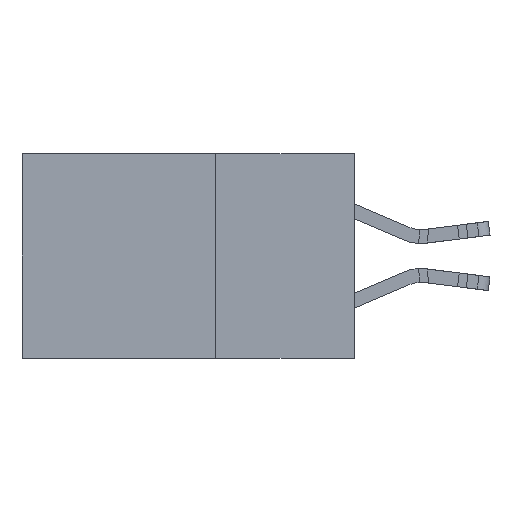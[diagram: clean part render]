
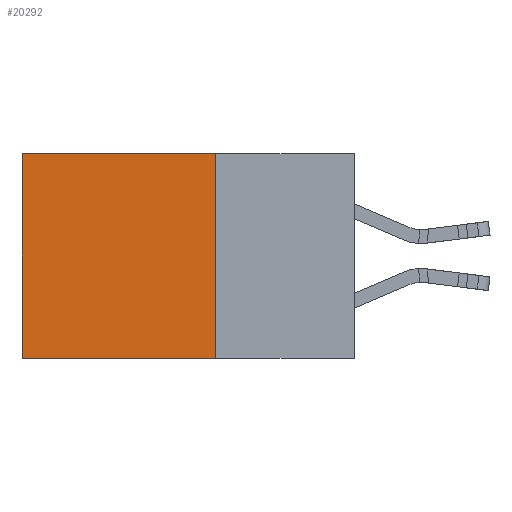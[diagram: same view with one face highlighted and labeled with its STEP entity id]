
A CAD part, left-side view. The second image highlights one B-rep face of the part: STEP entity #20292.
In plain terms, the highlighted planar face has unit normal (-1, 0, 0).
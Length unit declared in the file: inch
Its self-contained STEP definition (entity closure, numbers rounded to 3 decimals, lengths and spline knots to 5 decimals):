
#1641 = DIRECTION ( 'NONE',  ( 0., 1., 0. ) ) ;
#3402 = VERTEX_POINT ( 'NONE', #5823 ) ;
#4192 = EDGE_CURVE ( 'NONE', #12284, #3402, #6441, .T. ) ;
#5823 = CARTESIAN_POINT ( 'NONE',  ( 0.298, 0.6, 0. ) ) ;
#6295 = CARTESIAN_POINT ( 'NONE',  ( 0.298, 0.25, -0.37 ) ) ;
#6441 = LINE ( 'NONE', #18751, #32030 ) ;
#7421 = FACE_OUTER_BOUND ( 'NONE', #32267, .T. ) ;
#7775 = ORIENTED_EDGE ( 'NONE', *, *, #25204, .T. ) ;
#8091 = CARTESIAN_POINT ( 'NONE',  ( 0.298, 0.6, 0. ) ) ;
#9135 = LINE ( 'NONE', #23017, #14268 ) ;
#9235 = CARTESIAN_POINT ( 'NONE',  ( 0.298, 0.25, -0.37 ) ) ;
#10216 = ORIENTED_EDGE ( 'NONE', *, *, #21673, .F. ) ;
#10637 = DIRECTION ( 'NONE',  ( 0., 0., -1. ) ) ;
#11047 = DIRECTION ( 'NONE',  ( 0., 1., 0. ) ) ;
#12251 = VECTOR ( 'NONE', #10637, 39.37008 ) ;
#12284 = VERTEX_POINT ( 'NONE', #25795 ) ;
#12601 = PLANE ( 'NONE',  #14463 ) ;
#12894 = ORIENTED_EDGE ( 'NONE', *, *, #4192, .T. ) ;
#13270 = LINE ( 'NONE', #9235, #24955 ) ;
#13990 = VERTEX_POINT ( 'NONE', #29405 ) ;
#14268 = VECTOR ( 'NONE', #17965, 39.37008 ) ;
#14463 = AXIS2_PLACEMENT_3D ( 'NONE', #15029, #29901, #15143 ) ;
#15029 = CARTESIAN_POINT ( 'NONE',  ( 0.298, 0.25, 0. ) ) ;
#15143 = DIRECTION ( 'NONE',  ( 0., 0., -1. ) ) ;
#17965 = DIRECTION ( 'NONE',  ( 0., 0., -1. ) ) ;
#18751 = CARTESIAN_POINT ( 'NONE',  ( 0.298, 0.25, 0. ) ) ;
#20292 = ADVANCED_FACE ( 'NONE', ( #7421 ), #12601, .F. ) ;
#21673 = EDGE_CURVE ( 'NONE', #30632, #13990, #13270, .T. ) ;
#23017 = CARTESIAN_POINT ( 'NONE',  ( 0.298, 0.25, 0. ) ) ;
#24955 = VECTOR ( 'NONE', #1641, 39.37008 ) ;
#25204 = EDGE_CURVE ( 'NONE', #3402, #13990, #25517, .T. ) ;
#25517 = LINE ( 'NONE', #8091, #12251 ) ;
#25795 = CARTESIAN_POINT ( 'NONE',  ( 0.298, 0.25, 0. ) ) ;
#27000 = EDGE_CURVE ( 'NONE', #12284, #30632, #9135, .T. ) ;
#28837 = ORIENTED_EDGE ( 'NONE', *, *, #27000, .F. ) ;
#29405 = CARTESIAN_POINT ( 'NONE',  ( 0.298, 0.6, -0.37 ) ) ;
#29901 = DIRECTION ( 'NONE',  ( 1., 0., 0. ) ) ;
#30632 = VERTEX_POINT ( 'NONE', #6295 ) ;
#32030 = VECTOR ( 'NONE', #11047, 39.37008 ) ;
#32267 = EDGE_LOOP ( 'NONE', ( #7775, #10216, #28837, #12894 ) ) ;
